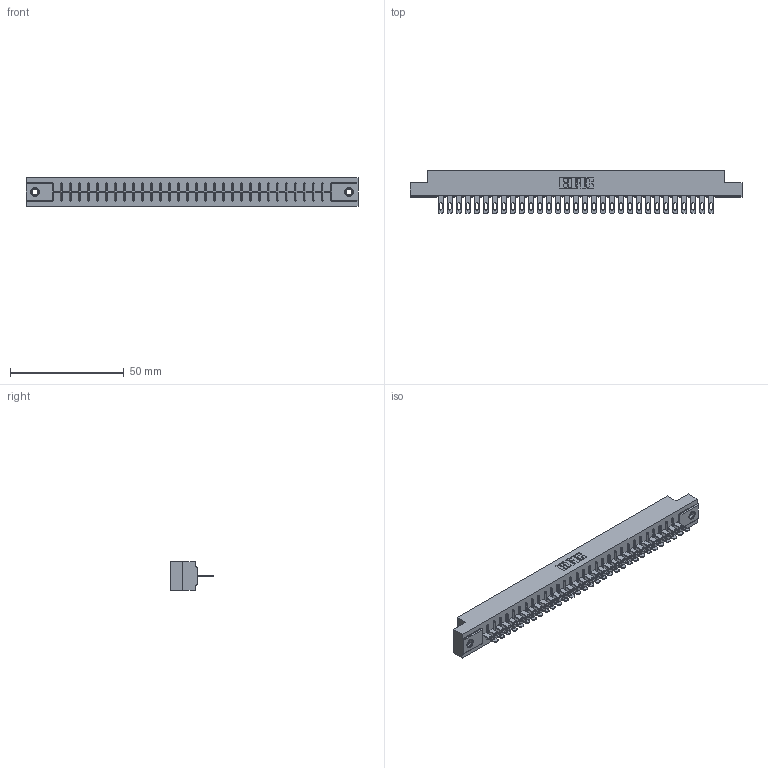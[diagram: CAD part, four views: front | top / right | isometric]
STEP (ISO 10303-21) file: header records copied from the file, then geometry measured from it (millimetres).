
FILE_DESCRIPTION (( 'STEP AP203' ), '1' );
FILE_NAME ('316-031-400-107.STEP', '2020-09-23T00:53:00', ( '' ), ( '' ), 'SwSTEP 2.0', 'SolidWorks 2020', '' );
FILE_SCHEMA (( 'CONFIG_CONTROL_DESIGN' ));
Length unit declared in the file: inch
Products named in the file (4): 306 Part_.156 Dia; 345-250-001_345-250-005-103; 316-031-400-107; 306-290-001_100
Assembly tree (34 placements, depth 2):
  316-031-400-107
    306 Part_.156 Dia
    306-290-001_100  x31
    345-250-001_345-250-005-103  x2
Bounding box: 145.85 x 18.87 x 12.7 mm (x, y, z)
Volume: 16120.2 mm3; surface area: 16996.6 mm2
Topology: 34 solids, 34 shells, 2532 faces, 7117 edges, 4570 vertices
Faces by surface type: plane 1650, cylinder 742, sphere 124, cone 12, torus 4
Entity records: 31683 total; most frequent: CARTESIAN_POINT 5299, ORIENTED_EDGE 5246, DIRECTION 5235, EDGE_CURVE 2623, LINE 2043, VECTOR 2043, VERTEX_POINT 1660, AXIS2_PLACEMENT_3D 1596
